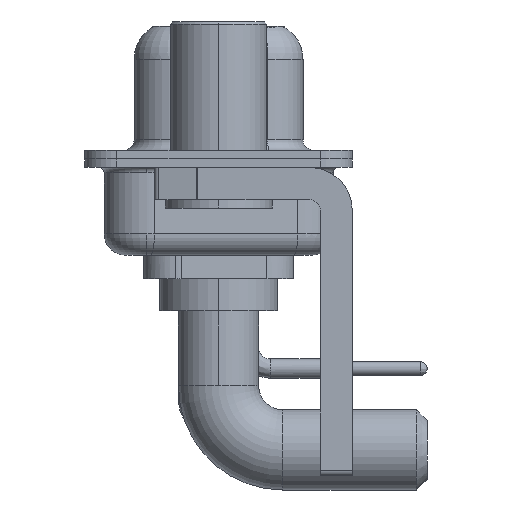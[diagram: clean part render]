
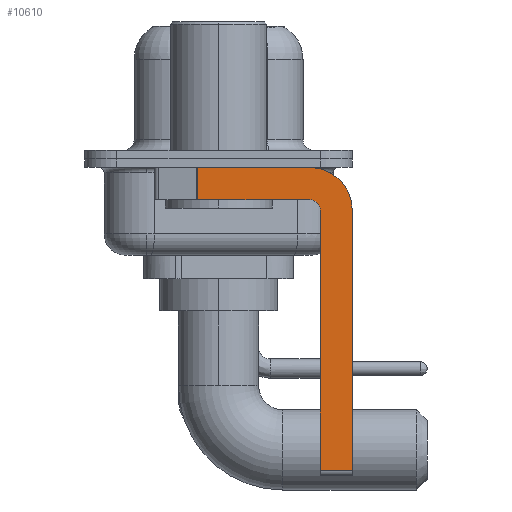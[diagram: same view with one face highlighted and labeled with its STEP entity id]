
A CAD part, left-side view. The second image highlights one B-rep face of the part: STEP entity #10610.
In plain terms, the highlighted planar face has unit normal (-1, 0, 0).
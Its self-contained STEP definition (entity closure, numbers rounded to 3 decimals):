
#29 = DIRECTION ( 'NONE',  ( 0., 0., -1. ) ) ;
#141 = VERTEX_POINT ( 'NONE', #9355 ) ;
#563 = VERTEX_POINT ( 'NONE', #15376 ) ;
#1069 = DIRECTION ( 'NONE',  ( -1., 0., 0. ) ) ;
#1322 = CARTESIAN_POINT ( 'NONE',  ( -2.9, -4.25, -2.4 ) ) ;
#1326 = VERTEX_POINT ( 'NONE', #17809 ) ;
#1999 = LINE ( 'NONE', #9546, #9231 ) ;
#2153 = DIRECTION ( 'NONE',  ( 0., 0., -1. ) ) ;
#2272 = PLANE ( 'NONE',  #13609 ) ;
#2427 = DIRECTION ( 'NONE',  ( 0., -1., 0. ) ) ;
#2778 = LINE ( 'NONE', #23263, #23505 ) ;
#3026 = AXIS2_PLACEMENT_3D ( 'NONE', #1322, #1069, #20166 ) ;
#3597 = DIRECTION ( 'NONE',  ( 0., 0., -1. ) ) ;
#4003 = CARTESIAN_POINT ( 'NONE',  ( -2.9, -4.25, -2.4 ) ) ;
#6071 = DIRECTION ( 'NONE',  ( 0., -1., 0. ) ) ;
#6823 = VECTOR ( 'NONE', #10567, 1000. ) ;
#6892 = EDGE_CURVE ( 'NONE', #1326, #13638, #7684, .T. ) ;
#7120 = CARTESIAN_POINT ( 'NONE',  ( -2.9, -6.25, -14.55 ) ) ;
#7676 = EDGE_CURVE ( 'NONE', #15990, #12843, #7768, .T. ) ;
#7684 = LINE ( 'NONE', #15262, #22098 ) ;
#7768 = CIRCLE ( 'NONE', #3026, 0.5 ) ;
#8182 = EDGE_CURVE ( 'NONE', #141, #20948, #2778, .T. ) ;
#9231 = VECTOR ( 'NONE', #6071, 1000. ) ;
#9355 = CARTESIAN_POINT ( 'NONE',  ( -2.9, -4.75, -14.55 ) ) ;
#9546 = CARTESIAN_POINT ( 'NONE',  ( -2.9, 3., -0.4 ) ) ;
#9830 = CARTESIAN_POINT ( 'NONE',  ( -2.9, -6.25, -2.4 ) ) ;
#9865 = EDGE_CURVE ( 'NONE', #563, #12387, #23116, .T. ) ;
#10347 = CARTESIAN_POINT ( 'NONE',  ( -2.9, -4.25, -1.9 ) ) ;
#10449 = CARTESIAN_POINT ( 'NONE',  ( -2.9, -4.75, -14.8 ) ) ;
#10567 = DIRECTION ( 'NONE',  ( 0., 0., 1. ) ) ;
#10610 = ADVANCED_FACE ( 'NONE', ( #17407 ), #2272, .F. ) ;
#10715 = LINE ( 'NONE', #10347, #17517 ) ;
#11082 = EDGE_CURVE ( 'NONE', #1326, #563, #1999, .T. ) ;
#11443 = LINE ( 'NONE', #9830, #18224 ) ;
#11491 = ORIENTED_EDGE ( 'NONE', *, *, #8182, .T. ) ;
#12220 = DIRECTION ( 'NONE',  ( 1., 0., 0. ) ) ;
#12387 = VERTEX_POINT ( 'NONE', #16894 ) ;
#12421 = CARTESIAN_POINT ( 'NONE',  ( -2.9, -4.75, -2.4 ) ) ;
#12843 = VERTEX_POINT ( 'NONE', #18347 ) ;
#13609 = AXIS2_PLACEMENT_3D ( 'NONE', #4003, #19007, #29 ) ;
#13638 = VERTEX_POINT ( 'NONE', #17597 ) ;
#13718 = ORIENTED_EDGE ( 'NONE', *, *, #6892, .T. ) ;
#14960 = ORIENTED_EDGE ( 'NONE', *, *, #22572, .F. ) ;
#15262 = CARTESIAN_POINT ( 'NONE',  ( -2.9, 0.978, -1.9 ) ) ;
#15376 = CARTESIAN_POINT ( 'NONE',  ( -2.9, -4.25, -0.4 ) ) ;
#15473 = ORIENTED_EDGE ( 'NONE', *, *, #7676, .F. ) ;
#15990 = VERTEX_POINT ( 'NONE', #12421 ) ;
#16894 = CARTESIAN_POINT ( 'NONE',  ( -2.9, -6.25, -2.4 ) ) ;
#17407 = FACE_OUTER_BOUND ( 'NONE', #17838, .T. ) ;
#17517 = VECTOR ( 'NONE', #18285, 1000. ) ;
#17597 = CARTESIAN_POINT ( 'NONE',  ( -2.9, 0.978, -1.9 ) ) ;
#17809 = CARTESIAN_POINT ( 'NONE',  ( -2.9, 0.978, -0.4 ) ) ;
#17838 = EDGE_LOOP ( 'NONE', ( #19802, #13718, #22445, #15473, #14960, #11491, #22970, #24174 ) ) ;
#18224 = VECTOR ( 'NONE', #2153, 1000. ) ;
#18285 = DIRECTION ( 'NONE',  ( 0., 1., 0. ) ) ;
#18347 = CARTESIAN_POINT ( 'NONE',  ( -2.9, -4.25, -1.9 ) ) ;
#19007 = DIRECTION ( 'NONE',  ( 1., 0., 0. ) ) ;
#19749 = EDGE_CURVE ( 'NONE', #12387, #20948, #11443, .T. ) ;
#19790 = DIRECTION ( 'NONE',  ( 0., 0., -1. ) ) ;
#19802 = ORIENTED_EDGE ( 'NONE', *, *, #11082, .F. ) ;
#19922 = AXIS2_PLACEMENT_3D ( 'NONE', #22019, #12220, #19790 ) ;
#20166 = DIRECTION ( 'NONE',  ( 0., 0., 1. ) ) ;
#20948 = VERTEX_POINT ( 'NONE', #7120 ) ;
#22019 = CARTESIAN_POINT ( 'NONE',  ( -2.9, -4.25, -2.4 ) ) ;
#22098 = VECTOR ( 'NONE', #3597, 1000. ) ;
#22183 = EDGE_CURVE ( 'NONE', #12843, #13638, #10715, .T. ) ;
#22445 = ORIENTED_EDGE ( 'NONE', *, *, #22183, .F. ) ;
#22572 = EDGE_CURVE ( 'NONE', #141, #15990, #23605, .T. ) ;
#22970 = ORIENTED_EDGE ( 'NONE', *, *, #19749, .F. ) ;
#23116 = CIRCLE ( 'NONE', #19922, 2. ) ;
#23263 = CARTESIAN_POINT ( 'NONE',  ( -2.9, -4.25, -14.55 ) ) ;
#23505 = VECTOR ( 'NONE', #2427, 1000. ) ;
#23605 = LINE ( 'NONE', #10449, #6823 ) ;
#24174 = ORIENTED_EDGE ( 'NONE', *, *, #9865, .F. ) ;
